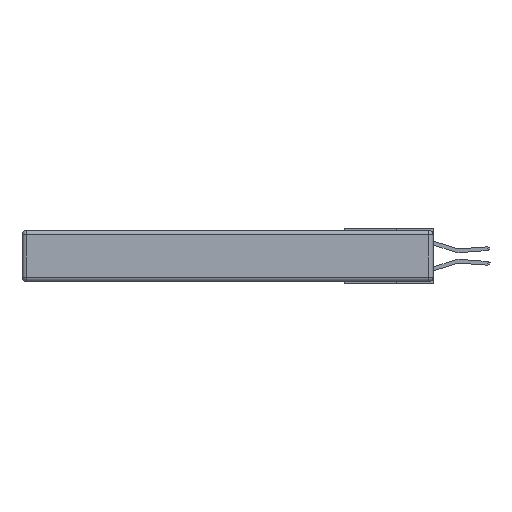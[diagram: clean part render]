
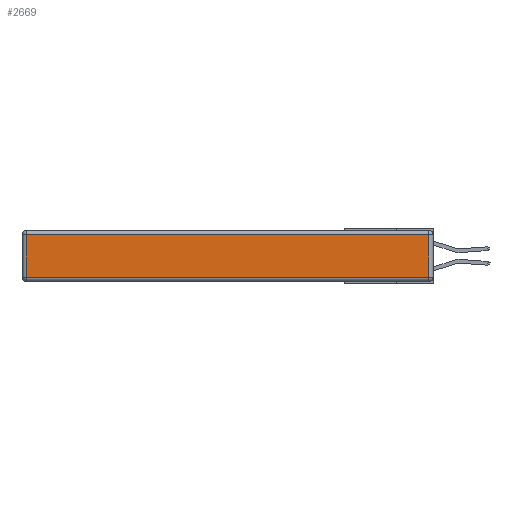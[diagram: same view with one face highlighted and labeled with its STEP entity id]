
A CAD part, left-side view. The second image highlights one B-rep face of the part: STEP entity #2669.
In plain terms, the highlighted planar face has unit normal (-1, 0, 0).
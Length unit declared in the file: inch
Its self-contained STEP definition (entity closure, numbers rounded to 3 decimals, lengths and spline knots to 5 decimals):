
#649 = ORIENTED_EDGE ( 'NONE', *, *, #834, .T. ) ;
#834 = EDGE_CURVE ( 'NONE', #17274, #4010, #11470, .T. ) ;
#1057 = EDGE_LOOP ( 'NONE', ( #9513, #649, #12799, #18794 ) ) ;
#1474 = DIRECTION ( 'NONE',  ( 0., 0., -1. ) ) ;
#1530 = CARTESIAN_POINT ( 'NONE',  ( 0., 2.72, -0.03 ) ) ;
#1699 = LINE ( 'NONE', #20465, #13626 ) ;
#2069 = EDGE_CURVE ( 'NONE', #5861, #12838, #1699, .T. ) ;
#2669 = ADVANCED_FACE ( 'NONE', ( #2906 ), #7804, .T. ) ;
#2906 = FACE_OUTER_BOUND ( 'NONE', #1057, .T. ) ;
#3894 = LINE ( 'NONE', #6750, #5634 ) ;
#4008 = EDGE_CURVE ( 'NONE', #12838, #17274, #14843, .T. ) ;
#4010 = VERTEX_POINT ( 'NONE', #4661 ) ;
#4661 = CARTESIAN_POINT ( 'NONE',  ( 0., 0.03, -0.03 ) ) ;
#4733 = EDGE_CURVE ( 'NONE', #4010, #5861, #3894, .T. ) ;
#5307 = DIRECTION ( 'NONE',  ( 0., 1., 0. ) ) ;
#5634 = VECTOR ( 'NONE', #5307, 39.37008 ) ;
#5807 = CARTESIAN_POINT ( 'NONE',  ( 0., 0., -0.313 ) ) ;
#5861 = VERTEX_POINT ( 'NONE', #1530 ) ;
#6750 = CARTESIAN_POINT ( 'NONE',  ( 0., 2.75, -0.03 ) ) ;
#7287 = CARTESIAN_POINT ( 'NONE',  ( 0., 0.03, -0.343 ) ) ;
#7608 = DIRECTION ( 'NONE',  ( -1., 0., 0. ) ) ;
#7804 = PLANE ( 'NONE',  #14313 ) ;
#9495 = DIRECTION ( 'NONE',  ( 0., -1., 0. ) ) ;
#9513 = ORIENTED_EDGE ( 'NONE', *, *, #4008, .T. ) ;
#11470 = LINE ( 'NONE', #7287, #19644 ) ;
#12799 = ORIENTED_EDGE ( 'NONE', *, *, #4733, .T. ) ;
#12838 = VERTEX_POINT ( 'NONE', #15903 ) ;
#13626 = VECTOR ( 'NONE', #1474, 39.37008 ) ;
#13740 = CARTESIAN_POINT ( 'NONE',  ( 0., 0.03, -0.313 ) ) ;
#13834 = VECTOR ( 'NONE', #9495, 39.37008 ) ;
#14313 = AXIS2_PLACEMENT_3D ( 'NONE', #17114, #7608, #18695 ) ;
#14843 = LINE ( 'NONE', #5807, #13834 ) ;
#15903 = CARTESIAN_POINT ( 'NONE',  ( 0., 2.72, -0.313 ) ) ;
#17114 = CARTESIAN_POINT ( 'NONE',  ( 0., 0., -0.343 ) ) ;
#17274 = VERTEX_POINT ( 'NONE', #13740 ) ;
#18695 = DIRECTION ( 'NONE',  ( 0., 0., 1. ) ) ;
#18794 = ORIENTED_EDGE ( 'NONE', *, *, #2069, .T. ) ;
#19644 = VECTOR ( 'NONE', #20111, 39.37008 ) ;
#20111 = DIRECTION ( 'NONE',  ( 0., 0., 1. ) ) ;
#20465 = CARTESIAN_POINT ( 'NONE',  ( 0., 2.72, -0.343 ) ) ;
